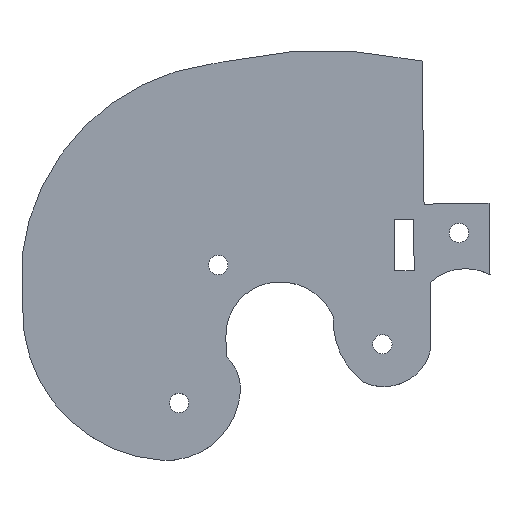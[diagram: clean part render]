
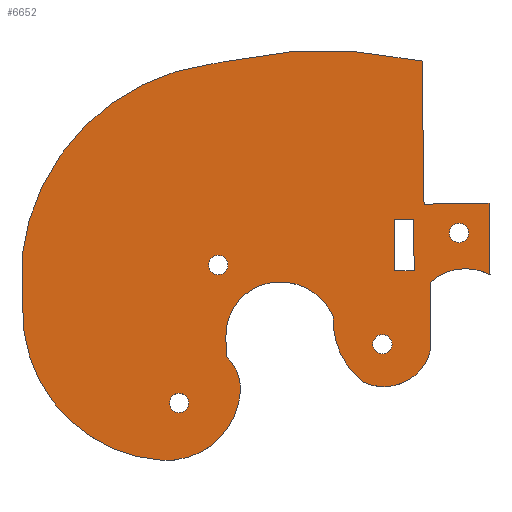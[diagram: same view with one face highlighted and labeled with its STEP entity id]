
A CAD part, top view. The second image highlights one B-rep face of the part: STEP entity #6652.
In plain terms, the highlighted planar face has unit normal (0, 0, 1).
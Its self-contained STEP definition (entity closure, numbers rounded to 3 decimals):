
#4526=CARTESIAN_POINT('',(27.37,7.001,10.0));
#4527=VERTEX_POINT('',#4526);
#4534=CARTESIAN_POINT('',(27.37,-0.999,10.0));
#4535=VERTEX_POINT('',#4534);
#4536=CARTESIAN_POINT('',(27.37,-0.999,10.0));
#4537=DIRECTION('',(0.0,1.0,0.0));
#4538=VECTOR('',#4537,8.0);
#4539=LINE('',#4536,#4538);
#4540=EDGE_CURVE('',#4535,#4527,#4539,.T.);
#4557=CARTESIAN_POINT('',(30.347,7.001,10.0));
#4558=VERTEX_POINT('',#4557);
#4565=CARTESIAN_POINT('',(27.37,7.001,10.0));
#4566=DIRECTION('',(1.0,0.0,0.0));
#4567=VECTOR('',#4566,2.977);
#4568=LINE('',#4565,#4567);
#4569=EDGE_CURVE('',#4527,#4558,#4568,.T.);
#4581=CARTESIAN_POINT('',(30.347,2.999,10.0));
#4582=VERTEX_POINT('',#4581);
#4589=CARTESIAN_POINT('',(30.347,7.001,10.0));
#4590=DIRECTION('',(0.0,-1.0,0.0));
#4591=VECTOR('',#4590,4.002);
#4592=LINE('',#4589,#4591);
#4593=EDGE_CURVE('',#4558,#4582,#4592,.T.);
#4605=CARTESIAN_POINT('',(30.458,-0.999,10.0));
#4606=VERTEX_POINT('',#4605);
#4613=CARTESIAN_POINT('',(30.347,2.999,10.0));
#4614=DIRECTION('',(0.028,-1.,0.0));
#4615=VECTOR('',#4614,4.);
#4616=LINE('',#4613,#4615);
#4617=EDGE_CURVE('',#4582,#4606,#4616,.T.);
#4630=CARTESIAN_POINT('',(30.458,-0.999,10.0));
#4631=DIRECTION('',(-1.0,0.0,0.0));
#4632=VECTOR('',#4631,3.088);
#4633=LINE('',#4630,#4632);
#4634=EDGE_CURVE('',#4606,#4535,#4633,.T.);
#6115=CARTESIAN_POINT('',(42.043,9.462,10.0));
#6116=VERTEX_POINT('',#6115);
#6123=CARTESIAN_POINT('',(42.197,-1.626,10.0));
#6124=VERTEX_POINT('',#6123);
#6125=CARTESIAN_POINT('',(42.043,9.462,10.0));
#6126=DIRECTION('',(0.014,-1.,0.0));
#6127=VECTOR('',#6126,11.089);
#6128=LINE('',#6125,#6127);
#6129=EDGE_CURVE('',#6116,#6124,#6128,.T.);
#6147=CARTESIAN_POINT('',(32.879,-2.836,10.0));
#6148=VERTEX_POINT('',#6147);
#6149=CARTESIAN_POINT('',(38.414,-8.974,10.0));
#6150=DIRECTION('',(0.0,0.0,1.0));
#6151=DIRECTION('',(0.458,0.889,0.0));
#6152=AXIS2_PLACEMENT_3D('',#6149,#6150,#6151);
#6153=CIRCLE('',#6152,8.265);
#6154=EDGE_CURVE('',#6124,#6148,#6153,.T.);
#6172=CARTESIAN_POINT('',(33.023,-13.137,10.0));
#6173=VERTEX_POINT('',#6172);
#6174=CARTESIAN_POINT('',(32.879,-2.836,10.0));
#6175=DIRECTION('',(0.014,-1.,0.0));
#6176=VECTOR('',#6175,10.302);
#6177=LINE('',#6174,#6176);
#6178=EDGE_CURVE('',#6148,#6173,#6177,.T.);
#6196=CARTESIAN_POINT('',(22.517,-18.329,10.0));
#6197=VERTEX_POINT('',#6196);
#6198=CARTESIAN_POINT('',(25.7,-11.545,10.0));
#6199=DIRECTION('',(0.0,0.0,-1.0));
#6200=DIRECTION('',(0.425,0.905,0.0));
#6201=AXIS2_PLACEMENT_3D('',#6198,#6199,#6200);
#6202=CIRCLE('',#6201,7.493);
#6203=EDGE_CURVE('',#6173,#6197,#6202,.T.);
#6221=CARTESIAN_POINT('',(17.879,-8.196,10.0));
#6222=VERTEX_POINT('',#6221);
#6223=CARTESIAN_POINT('',(29.931,-8.807,10.0));
#6224=DIRECTION('',(0.0,0.0,-1.0));
#6225=DIRECTION('',(0.999,-0.051,0.0));
#6226=AXIS2_PLACEMENT_3D('',#6223,#6224,#6225);
#6227=CIRCLE('',#6226,12.068);
#6228=EDGE_CURVE('',#6197,#6222,#6227,.T.);
#6246=CARTESIAN_POINT('',(9.147,-2.786,10.0));
#6247=VERTEX_POINT('',#6246);
#6248=CARTESIAN_POINT('',(9.645,-11.733,10.0));
#6249=DIRECTION('',(0.0,0.0,1.0));
#6250=DIRECTION('',(0.919,0.395,0.0));
#6251=AXIS2_PLACEMENT_3D('',#6248,#6249,#6250);
#6252=CIRCLE('',#6251,8.962);
#6253=EDGE_CURVE('',#6222,#6247,#6252,.T.);
#6271=CARTESIAN_POINT('',(1.183,-11.177,10.0));
#6272=VERTEX_POINT('',#6271);
#6273=CARTESIAN_POINT('',(9.465,-11.062,10.0));
#6274=DIRECTION('',(0.0,0.0,1.0));
#6275=DIRECTION('',(-0.038,0.999,0.0));
#6276=AXIS2_PLACEMENT_3D('',#6273,#6274,#6275);
#6277=CIRCLE('',#6276,8.283);
#6278=EDGE_CURVE('',#6247,#6272,#6277,.T.);
#6296=CARTESIAN_POINT('',(1.227,-14.344,10.0));
#6297=VERTEX_POINT('',#6296);
#6298=CARTESIAN_POINT('',(1.183,-11.177,10.0));
#6299=DIRECTION('',(0.014,-1.,0.0));
#6300=VECTOR('',#6299,3.167);
#6301=LINE('',#6298,#6300);
#6302=EDGE_CURVE('',#6272,#6297,#6301,.T.);
#6320=CARTESIAN_POINT('',(3.421,-19.791,10.0));
#6321=VERTEX_POINT('',#6320);
#6322=CARTESIAN_POINT('',(-3.3,-19.333,10.0));
#6323=DIRECTION('',(0.0,0.0,-1.0));
#6324=DIRECTION('',(-0.998,0.068,0.0));
#6325=AXIS2_PLACEMENT_3D('',#6322,#6323,#6324);
#6326=CIRCLE('',#6325,6.737);
#6327=EDGE_CURVE('',#6297,#6321,#6326,.T.);
#6345=CARTESIAN_POINT('',(-8.785,-30.458,10.0));
#6346=VERTEX_POINT('',#6345);
#6347=CARTESIAN_POINT('',(-8.025,-19.011,10.0));
#6348=DIRECTION('',(0.0,0.0,-1.0));
#6349=DIRECTION('',(0.066,0.998,0.0));
#6350=AXIS2_PLACEMENT_3D('',#6347,#6348,#6349);
#6351=CIRCLE('',#6350,11.473);
#6352=EDGE_CURVE('',#6321,#6346,#6351,.T.);
#6370=CARTESIAN_POINT('',(-30.377,-6.647,10.0));
#6371=VERTEX_POINT('',#6370);
#6372=CARTESIAN_POINT('',(-7.252,-7.373,10.0));
#6373=DIRECTION('',(0.0,0.0,-1.0));
#6374=DIRECTION('',(1.,-0.031,0.0));
#6375=AXIS2_PLACEMENT_3D('',#6372,#6373,#6374);
#6376=CIRCLE('',#6375,23.137);
#6377=EDGE_CURVE('',#6346,#6371,#6376,.T.);
#6395=CARTESIAN_POINT('',(-30.488,1.29,10.0));
#6396=VERTEX_POINT('',#6395);
#6397=CARTESIAN_POINT('',(-30.377,-6.647,10.0));
#6398=DIRECTION('',(-0.014,1.,0.0));
#6399=VECTOR('',#6398,7.938);
#6400=LINE('',#6397,#6399);
#6401=EDGE_CURVE('',#6371,#6396,#6400,.T.);
#6419=CARTESIAN_POINT('',(-1.045,31.105,10.0));
#6420=VERTEX_POINT('',#6419);
#6421=CARTESIAN_POINT('',(3.33,-2.659,10.0));
#6422=DIRECTION('',(0.0,0.0,-1.0));
#6423=DIRECTION('',(0.128,-0.992,0.0));
#6424=AXIS2_PLACEMENT_3D('',#6421,#6422,#6423);
#6425=CIRCLE('',#6424,34.047);
#6426=EDGE_CURVE('',#6396,#6420,#6425,.T.);
#6444=CARTESIAN_POINT('',(0.746,31.421,10.0));
#6445=VERTEX_POINT('',#6444);
#6446=CARTESIAN_POINT('',(-3.614,50.94,10.0));
#6447=DIRECTION('',(0.0,0.0,1.0));
#6448=DIRECTION('',(0.128,-0.992,0.0));
#6449=AXIS2_PLACEMENT_3D('',#6446,#6447,#6448);
#6450=CIRCLE('',#6449,20.0);
#6451=EDGE_CURVE('',#6420,#6445,#6450,.T.);
#6469=CARTESIAN_POINT('',(31.643,31.541,10.0));
#6470=VERTEX_POINT('',#6469);
#6471=CARTESIAN_POINT('',(16.469,-38.968,10.0));
#6472=DIRECTION('',(0.0,0.0,-1.0));
#6473=DIRECTION('',(-0.21,-0.978,0.0));
#6474=AXIS2_PLACEMENT_3D('',#6471,#6472,#6473);
#6475=CIRCLE('',#6474,72.123);
#6476=EDGE_CURVE('',#6445,#6470,#6475,.T.);
#6495=CARTESIAN_POINT('',(38.881,4.849,10.0));
#6496=VERTEX_POINT('',#6495);
#6497=CARTESIAN_POINT('',(37.381,4.849,10.0));
#6498=DIRECTION('',(0.0,0.0,1.0));
#6499=DIRECTION('',(-1.0,0.0,0.0));
#6500=AXIS2_PLACEMENT_3D('',#6497,#6498,#6499);
#6501=CIRCLE('',#6500,1.5);
#6502=EDGE_CURVE('',#6496,#6496,#6501,.T.);
#6515=CARTESIAN_POINT('',(26.997,-12.439,10.0));
#6516=VERTEX_POINT('',#6515);
#6517=CARTESIAN_POINT('',(25.497,-12.439,10.0));
#6518=DIRECTION('',(0.0,0.0,1.0));
#6519=DIRECTION('',(-1.0,0.0,0.0));
#6520=AXIS2_PLACEMENT_3D('',#6517,#6518,#6519);
#6521=CIRCLE('',#6520,1.5);
#6522=EDGE_CURVE('',#6516,#6516,#6521,.T.);
#6535=CARTESIAN_POINT('',(1.49,-0.126,10.0));
#6536=VERTEX_POINT('',#6535);
#6537=CARTESIAN_POINT('',(-0.01,-0.126,10.0));
#6538=DIRECTION('',(0.0,0.0,1.0));
#6539=DIRECTION('',(-1.0,0.0,0.0));
#6540=AXIS2_PLACEMENT_3D('',#6537,#6538,#6539);
#6541=CIRCLE('',#6540,1.5);
#6542=EDGE_CURVE('',#6536,#6536,#6541,.T.);
#6555=CARTESIAN_POINT('',(-4.58,-21.577,10.0));
#6556=VERTEX_POINT('',#6555);
#6557=CARTESIAN_POINT('',(-6.08,-21.577,10.0));
#6558=DIRECTION('',(0.0,0.0,1.0));
#6559=DIRECTION('',(-1.0,0.0,0.0));
#6560=AXIS2_PLACEMENT_3D('',#6557,#6558,#6559);
#6561=CIRCLE('',#6560,1.5);
#6562=EDGE_CURVE('',#6556,#6556,#6561,.T.);
#6574=CARTESIAN_POINT('',(31.952,9.322,10.0));
#6575=VERTEX_POINT('',#6574);
#6576=CARTESIAN_POINT('',(31.643,31.541,10.0));
#6577=DIRECTION('',(0.014,-1.,0.0));
#6578=VECTOR('',#6577,22.222);
#6579=LINE('',#6576,#6578);
#6580=EDGE_CURVE('',#6470,#6575,#6579,.T.);
#6597=CARTESIAN_POINT('',(31.952,9.322,10.0));
#6598=DIRECTION('',(1.,0.014,0.0));
#6599=VECTOR('',#6598,10.092);
#6600=LINE('',#6597,#6599);
#6601=EDGE_CURVE('',#6575,#6116,#6600,.T.);
#6609=CARTESIAN_POINT('',(7.819,2.386,10.0));
#6610=DIRECTION('',(0.0,0.0,1.0));
#6611=DIRECTION('',(1.0,0.0,0.0));
#6612=AXIS2_PLACEMENT_3D('',#6609,#6610,#6611);
#6613=PLANE('',#6612);
#6614=ORIENTED_EDGE('',*,*,#6601,.F.);
#6615=ORIENTED_EDGE('',*,*,#6580,.F.);
#6616=ORIENTED_EDGE('',*,*,#6476,.F.);
#6617=ORIENTED_EDGE('',*,*,#6451,.F.);
#6618=ORIENTED_EDGE('',*,*,#6426,.F.);
#6619=ORIENTED_EDGE('',*,*,#6401,.F.);
#6620=ORIENTED_EDGE('',*,*,#6377,.F.);
#6621=ORIENTED_EDGE('',*,*,#6352,.F.);
#6622=ORIENTED_EDGE('',*,*,#6327,.F.);
#6623=ORIENTED_EDGE('',*,*,#6302,.F.);
#6624=ORIENTED_EDGE('',*,*,#6278,.F.);
#6625=ORIENTED_EDGE('',*,*,#6253,.F.);
#6626=ORIENTED_EDGE('',*,*,#6228,.F.);
#6627=ORIENTED_EDGE('',*,*,#6203,.F.);
#6628=ORIENTED_EDGE('',*,*,#6178,.F.);
#6629=ORIENTED_EDGE('',*,*,#6154,.F.);
#6630=ORIENTED_EDGE('',*,*,#6129,.F.);
#6631=EDGE_LOOP('',(#6614,#6615,#6616,#6617,#6618,#6619,#6620,#6621,#6622,#6623,#6624,#6625,#6626,#6627,#6628,#6629,#6630));
#6632=FACE_OUTER_BOUND('',#6631,.T.);
#6633=ORIENTED_EDGE('',*,*,#4540,.T.);
#6634=ORIENTED_EDGE('',*,*,#4569,.T.);
#6635=ORIENTED_EDGE('',*,*,#4593,.T.);
#6636=ORIENTED_EDGE('',*,*,#4617,.T.);
#6637=ORIENTED_EDGE('',*,*,#4634,.T.);
#6638=EDGE_LOOP('',(#6633,#6634,#6635,#6636,#6637));
#6639=FACE_BOUND('',#6638,.T.);
#6640=ORIENTED_EDGE('',*,*,#6502,.F.);
#6641=EDGE_LOOP('',(#6640));
#6642=FACE_BOUND('',#6641,.T.);
#6643=ORIENTED_EDGE('',*,*,#6522,.F.);
#6644=EDGE_LOOP('',(#6643));
#6645=FACE_BOUND('',#6644,.T.);
#6646=ORIENTED_EDGE('',*,*,#6542,.F.);
#6647=EDGE_LOOP('',(#6646));
#6648=FACE_BOUND('',#6647,.T.);
#6649=ORIENTED_EDGE('',*,*,#6562,.F.);
#6650=EDGE_LOOP('',(#6649));
#6651=FACE_BOUND('',#6650,.T.);
#6652=ADVANCED_FACE('',(#6632,#6639,#6642,#6645,#6648,#6651),#6613,.T.);
